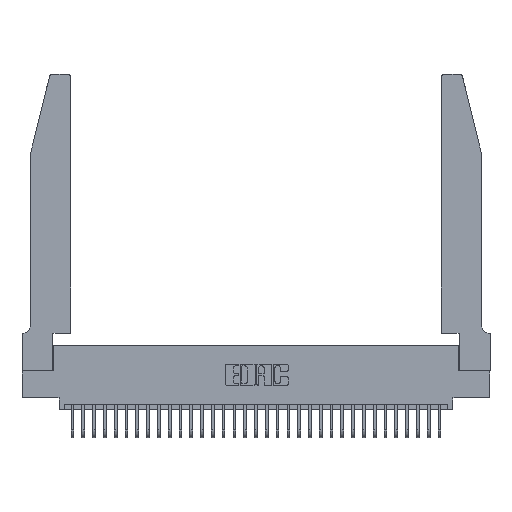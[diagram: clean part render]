
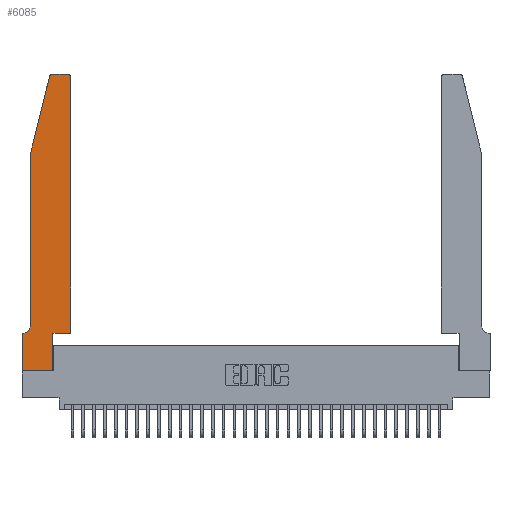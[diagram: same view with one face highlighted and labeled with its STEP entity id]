
A CAD part, top view. The second image highlights one B-rep face of the part: STEP entity #6085.
In plain terms, the highlighted planar face has unit normal (0, 0, 1).
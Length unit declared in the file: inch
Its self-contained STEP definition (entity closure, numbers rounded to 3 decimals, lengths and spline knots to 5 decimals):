
#93 = CARTESIAN_POINT ( 'NONE',  ( 0.0755, 0.35, 0.37 ) ) ;
#1122 = VECTOR ( 'NONE', #18492, 39.37008 ) ;
#1296 = EDGE_CURVE ( 'NONE', #33273, #25747, #21584, .T. ) ;
#3077 = VERTEX_POINT ( 'NONE', #26185 ) ;
#3105 = EDGE_CURVE ( 'NONE', #5882, #32877, #31614, .T. ) ;
#3266 = AXIS2_PLACEMENT_3D ( 'NONE', #8195, #32200, #29214 ) ;
#3673 = CARTESIAN_POINT ( 'NONE',  ( 0.4505, 0.35, 0.37 ) ) ;
#3757 = CIRCLE ( 'NONE', #10920, 0.07 ) ;
#4247 = DIRECTION ( 'NONE',  ( 0., 1., 0. ) ) ;
#4304 = CARTESIAN_POINT ( 'NONE',  ( 0.0755, 2., 0.37 ) ) ;
#4912 = LINE ( 'NONE', #32135, #1122 ) ;
#5377 = CARTESIAN_POINT ( 'NONE',  ( 0.284, 2.72, 0.37 ) ) ;
#5584 = PLANE ( 'NONE',  #3266 ) ;
#5882 = VERTEX_POINT ( 'NONE', #31153 ) ;
#6085 = ADVANCED_FACE ( 'NONE', ( #11569 ), #5584, .T. ) ;
#6118 = DIRECTION ( 'NONE',  ( 0., 0., 1. ) ) ;
#6208 = DIRECTION ( 'NONE',  ( 0., -1., 0. ) ) ;
#7100 = VECTOR ( 'NONE', #31037, 39.37008 ) ;
#7255 = LINE ( 'NONE', #28097, #17796 ) ;
#7947 = EDGE_CURVE ( 'NONE', #32877, #27654, #28783, .T. ) ;
#7980 = DIRECTION ( 'NONE',  ( -1., 0., 0. ) ) ;
#8005 = DIRECTION ( 'NONE',  ( 1., 0., 0. ) ) ;
#8195 = CARTESIAN_POINT ( 'NONE',  ( 0., 0.35, 0.37 ) ) ;
#8427 = AXIS2_PLACEMENT_3D ( 'NONE', #22387, #6118, #22046 ) ;
#9236 = EDGE_CURVE ( 'NONE', #11396, #25789, #19273, .T. ) ;
#9980 = EDGE_CURVE ( 'NONE', #21099, #11396, #4912, .T. ) ;
#9991 = ORIENTED_EDGE ( 'NONE', *, *, #29753, .T. ) ;
#10920 = AXIS2_PLACEMENT_3D ( 'NONE', #15990, #26942, #29790 ) ;
#11396 = VERTEX_POINT ( 'NONE', #26888 ) ;
#11569 = FACE_OUTER_BOUND ( 'NONE', #32633, .T. ) ;
#12057 = ORIENTED_EDGE ( 'NONE', *, *, #30623, .T. ) ;
#13711 = CARTESIAN_POINT ( 'NONE',  ( 0.4505, 0.35, 0.37 ) ) ;
#14342 = VECTOR ( 'NONE', #19166, 39.37008 ) ;
#15285 = ORIENTED_EDGE ( 'NONE', *, *, #33757, .T. ) ;
#15704 = ORIENTED_EDGE ( 'NONE', *, *, #3105, .T. ) ;
#15990 = CARTESIAN_POINT ( 'NONE',  ( 0.0055, 0.42, 0.37 ) ) ;
#16077 = CARTESIAN_POINT ( 'NONE',  ( 0., 0.35, 0.37 ) ) ;
#16269 = CARTESIAN_POINT ( 'NONE',  ( 0.0755, 2., 0.37 ) ) ;
#16332 = ORIENTED_EDGE ( 'NONE', *, *, #9236, .T. ) ;
#16683 = LINE ( 'NONE', #4304, #23030 ) ;
#17153 = CARTESIAN_POINT ( 'NONE',  ( 0., 0., 0.37 ) ) ;
#17498 = VECTOR ( 'NONE', #4247, 39.37008 ) ;
#17796 = VECTOR ( 'NONE', #17968, 39.37008 ) ;
#17968 = DIRECTION ( 'NONE',  ( 1., 0., 0. ) ) ;
#18019 = VECTOR ( 'NONE', #22877, 39.37008 ) ;
#18492 = DIRECTION ( 'NONE',  ( 0., 1., 0. ) ) ;
#19166 = DIRECTION ( 'NONE',  ( 0., -1., 0. ) ) ;
#19273 = LINE ( 'NONE', #28893, #18019 ) ;
#19397 = CARTESIAN_POINT ( 'NONE',  ( 0., 0., 0.37 ) ) ;
#20463 = EDGE_CURVE ( 'NONE', #3077, #25397, #32370, .T. ) ;
#20473 = LINE ( 'NONE', #13711, #17498 ) ;
#21099 = VERTEX_POINT ( 'NONE', #29883 ) ;
#21374 = ORIENTED_EDGE ( 'NONE', *, *, #9980, .T. ) ;
#21412 = ORIENTED_EDGE ( 'NONE', *, *, #24036, .T. ) ;
#21584 = LINE ( 'NONE', #16269, #14342 ) ;
#21649 = VERTEX_POINT ( 'NONE', #29384 ) ;
#22046 = DIRECTION ( 'NONE',  ( 1., 0., 0. ) ) ;
#22322 = VERTEX_POINT ( 'NONE', #25088 ) ;
#22387 = CARTESIAN_POINT ( 'NONE',  ( 0.4205, 2.72, 0.37 ) ) ;
#22559 = ORIENTED_EDGE ( 'NONE', *, *, #32850, .T. ) ;
#22877 = DIRECTION ( 'NONE',  ( 1., 0., 0. ) ) ;
#22913 = ORIENTED_EDGE ( 'NONE', *, *, #20463, .T. ) ;
#23030 = VECTOR ( 'NONE', #33989, 39.37008 ) ;
#24036 = EDGE_CURVE ( 'NONE', #25789, #3077, #20473, .T. ) ;
#24138 = DIRECTION ( 'NONE',  ( 0., 0., 1. ) ) ;
#24754 = CARTESIAN_POINT ( 'NONE',  ( 0.0755, 0.42, 0.37 ) ) ;
#25088 = CARTESIAN_POINT ( 'NONE',  ( 0.284, 2.75, 0.37 ) ) ;
#25397 = VERTEX_POINT ( 'NONE', #33402 ) ;
#25747 = VERTEX_POINT ( 'NONE', #24754 ) ;
#25789 = VERTEX_POINT ( 'NONE', #3673 ) ;
#25974 = ORIENTED_EDGE ( 'NONE', *, *, #34074, .T. ) ;
#25996 = VECTOR ( 'NONE', #7980, 39.37008 ) ;
#26185 = CARTESIAN_POINT ( 'NONE',  ( 0.4505, 2.72, 0.37 ) ) ;
#26491 = ORIENTED_EDGE ( 'NONE', *, *, #1296, .T. ) ;
#26888 = CARTESIAN_POINT ( 'NONE',  ( 0.2865, 0.35, 0.37 ) ) ;
#26942 = DIRECTION ( 'NONE',  ( 0., 0., -1. ) ) ;
#27654 = VERTEX_POINT ( 'NONE', #19397 ) ;
#28097 = CARTESIAN_POINT ( 'NONE',  ( 0., 0., 0.37 ) ) ;
#28703 = AXIS2_PLACEMENT_3D ( 'NONE', #5377, #24138, #8005 ) ;
#28783 = LINE ( 'NONE', #17153, #29606 ) ;
#28893 = CARTESIAN_POINT ( 'NONE',  ( 0.4505, 0.35, 0.37 ) ) ;
#29214 = DIRECTION ( 'NONE',  ( 1., 0., 0. ) ) ;
#29384 = CARTESIAN_POINT ( 'NONE',  ( 0.25487, 2.72718, 0.37 ) ) ;
#29606 = VECTOR ( 'NONE', #6208, 39.37008 ) ;
#29753 = EDGE_CURVE ( 'NONE', #27654, #21099, #7255, .T. ) ;
#29790 = DIRECTION ( 'NONE',  ( -1., 0., 0. ) ) ;
#29883 = CARTESIAN_POINT ( 'NONE',  ( 0.2865, 0., 0.37 ) ) ;
#30623 = EDGE_CURVE ( 'NONE', #25747, #5882, #3757, .T. ) ;
#31037 = DIRECTION ( 'NONE',  ( -1., 0., 0. ) ) ;
#31153 = CARTESIAN_POINT ( 'NONE',  ( 0.0055, 0.35, 0.37 ) ) ;
#31399 = ORIENTED_EDGE ( 'NONE', *, *, #7947, .T. ) ;
#31614 = LINE ( 'NONE', #93, #7100 ) ;
#32135 = CARTESIAN_POINT ( 'NONE',  ( 0.2865, 0.35, 0.37 ) ) ;
#32200 = DIRECTION ( 'NONE',  ( 0., 0., 1. ) ) ;
#32268 = CARTESIAN_POINT ( 'NONE',  ( 0.0755, 2., 0.37 ) ) ;
#32370 = CIRCLE ( 'NONE', #8427, 0.03 ) ;
#32443 = CARTESIAN_POINT ( 'NONE',  ( 0.2605, 2.75, 0.37 ) ) ;
#32633 = EDGE_LOOP ( 'NONE', ( #25974, #22559, #15285, #26491, #12057, #15704, #31399, #9991, #21374, #16332, #21412, #22913 ) ) ;
#32850 = EDGE_CURVE ( 'NONE', #22322, #21649, #33258, .T. ) ;
#32877 = VERTEX_POINT ( 'NONE', #16077 ) ;
#33258 = CIRCLE ( 'NONE', #28703, 0.03 ) ;
#33273 = VERTEX_POINT ( 'NONE', #32268 ) ;
#33402 = CARTESIAN_POINT ( 'NONE',  ( 0.4205, 2.75, 0.37 ) ) ;
#33757 = EDGE_CURVE ( 'NONE', #21649, #33273, #16683, .T. ) ;
#33989 = DIRECTION ( 'NONE',  ( -0.239, -0.971, 0. ) ) ;
#34026 = LINE ( 'NONE', #32443, #25996 ) ;
#34074 = EDGE_CURVE ( 'NONE', #25397, #22322, #34026, .T. ) ;
